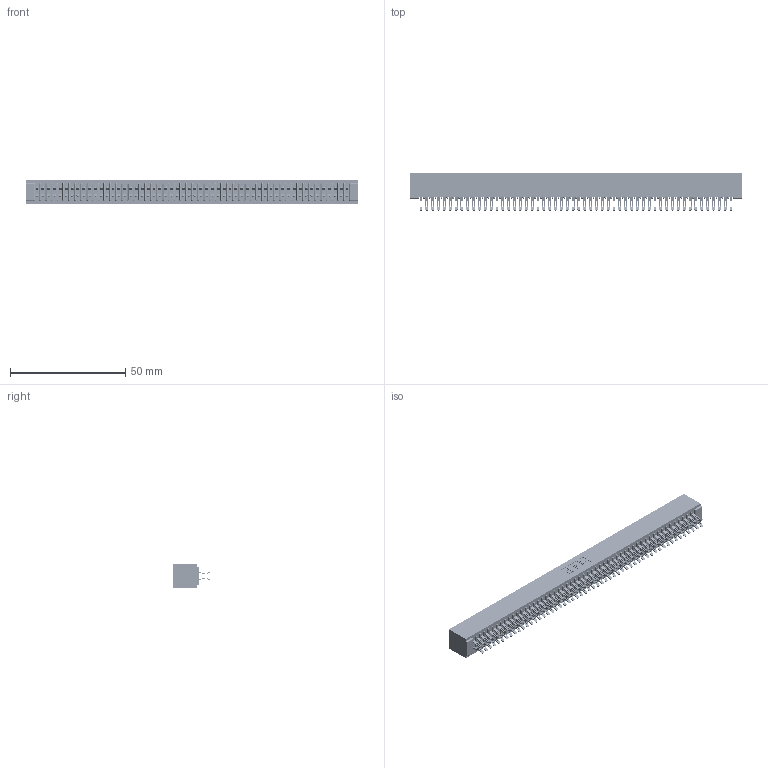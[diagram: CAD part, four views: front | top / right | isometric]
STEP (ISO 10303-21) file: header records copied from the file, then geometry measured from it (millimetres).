
FILE_DESCRIPTION (( 'STEP AP203' ), '1' );
FILE_NAME ('341-108-555-201.STEP', '2018-08-08T12:23:26', ( '' ), ( '' ), 'SwSTEP 2.0', 'SolidWorks 2016', '' );
FILE_SCHEMA (( 'CONFIG_CONTROL_DESIGN' ));
Length unit declared in the file: inch
Products named in the file (3): 341-292-001_341-292-155; 341-108-555-201; 341 Part_No Mounting Lugs
Assembly tree (109 placements, depth 2):
  341-108-555-201
    341 Part_No Mounting Lugs
    341-292-001_341-292-155  x108
Bounding box: 144.15 x 16.31 x 10.16 mm (x, y, z)
Volume: 11028.1 mm3; surface area: 21498.7 mm2
Topology: 109 solids, 109 shells, 8532 faces, 25510 edges, 16606 vertices
Faces by surface type: plane 4600, cylinder 3716, sphere 110, torus 106
Entity records: 63945 total; most frequent: CARTESIAN_POINT 10644, ORIENTED_EDGE 10568, DIRECTION 10310, EDGE_CURVE 5284, LINE 4270, VECTOR 4270, VERTEX_POINT 3338, AXIS2_PLACEMENT_3D 3020
